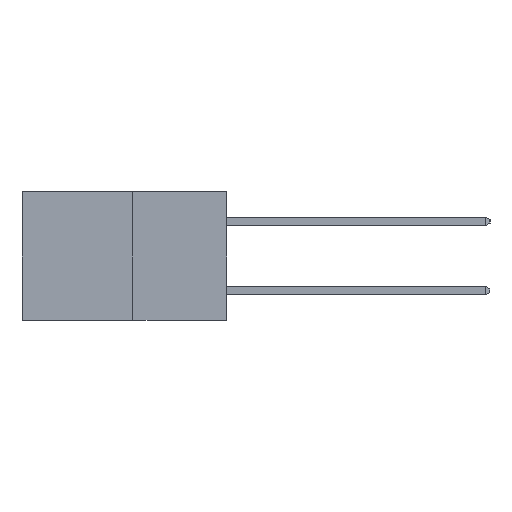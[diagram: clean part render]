
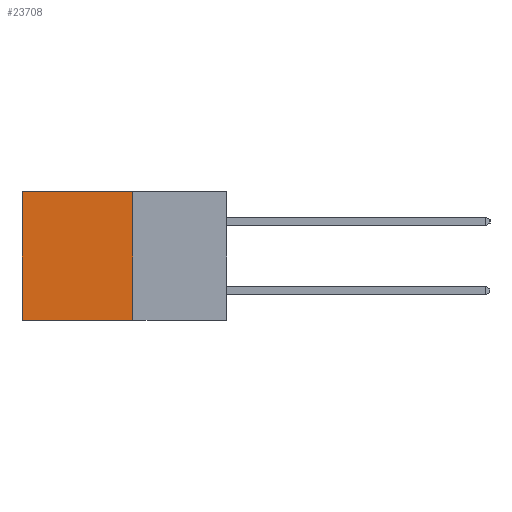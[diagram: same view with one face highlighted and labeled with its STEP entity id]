
A CAD part, left-side view. The second image highlights one B-rep face of the part: STEP entity #23708.
In plain terms, the highlighted planar face has unit normal (-1, 0, 0).
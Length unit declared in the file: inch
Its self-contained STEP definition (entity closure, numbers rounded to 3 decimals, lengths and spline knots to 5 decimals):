
#586 = CARTESIAN_POINT ( 'NONE',  ( 0.277, 0.27, -0.37 ) ) ;
#1063 = DIRECTION ( 'NONE',  ( 0., 1., 0. ) ) ;
#1952 = EDGE_CURVE ( 'NONE', #17042, #14268, #21985, .T. ) ;
#2075 = DIRECTION ( 'NONE',  ( 0., 0., -1. ) ) ;
#2226 = CARTESIAN_POINT ( 'NONE',  ( 0.277, 0.59, -0.37 ) ) ;
#4217 = LINE ( 'NONE', #586, #15182 ) ;
#5504 = EDGE_CURVE ( 'NONE', #17709, #29185, #4217, .T. ) ;
#5731 = CARTESIAN_POINT ( 'NONE',  ( 0.277, 0.27, -0.37 ) ) ;
#6723 = LINE ( 'NONE', #15952, #24613 ) ;
#8320 = CARTESIAN_POINT ( 'NONE',  ( 0.277, 0.59, 0. ) ) ;
#8503 = DIRECTION ( 'NONE',  ( 0., 1., 0. ) ) ;
#9946 = ORIENTED_EDGE ( 'NONE', *, *, #19311, .F. ) ;
#10320 = ORIENTED_EDGE ( 'NONE', *, *, #27218, .T. ) ;
#11307 = CARTESIAN_POINT ( 'NONE',  ( 0.277, 0.27, 0. ) ) ;
#13585 = CARTESIAN_POINT ( 'NONE',  ( 0.277, 0.27, -0.37 ) ) ;
#13895 = AXIS2_PLACEMENT_3D ( 'NONE', #13585, #16037, #2075 ) ;
#14268 = VERTEX_POINT ( 'NONE', #8320 ) ;
#15182 = VECTOR ( 'NONE', #1063, 39.37008 ) ;
#15952 = CARTESIAN_POINT ( 'NONE',  ( 0.277, 0.27, -0.37 ) ) ;
#16037 = DIRECTION ( 'NONE',  ( 1., 0., 0. ) ) ;
#17042 = VERTEX_POINT ( 'NONE', #11307 ) ;
#17619 = EDGE_LOOP ( 'NONE', ( #10320, #29735, #9946, #27621 ) ) ;
#17709 = VERTEX_POINT ( 'NONE', #5731 ) ;
#18183 = LINE ( 'NONE', #2226, #18936 ) ;
#18804 = CARTESIAN_POINT ( 'NONE',  ( 0.277, 0.59, -0.37 ) ) ;
#18936 = VECTOR ( 'NONE', #27805, 39.37008 ) ;
#19311 = EDGE_CURVE ( 'NONE', #17042, #17709, #6723, .T. ) ;
#20399 = CARTESIAN_POINT ( 'NONE',  ( 0.277, 0.27, 0. ) ) ;
#20494 = VECTOR ( 'NONE', #8503, 39.37008 ) ;
#21985 = LINE ( 'NONE', #20399, #20494 ) ;
#23708 = ADVANCED_FACE ( 'NONE', ( #26323 ), #25277, .F. ) ;
#24613 = VECTOR ( 'NONE', #29854, 39.37008 ) ;
#25277 = PLANE ( 'NONE',  #13895 ) ;
#26323 = FACE_OUTER_BOUND ( 'NONE', #17619, .T. ) ;
#27218 = EDGE_CURVE ( 'NONE', #14268, #29185, #18183, .T. ) ;
#27621 = ORIENTED_EDGE ( 'NONE', *, *, #1952, .T. ) ;
#27805 = DIRECTION ( 'NONE',  ( 0., 0., -1. ) ) ;
#29185 = VERTEX_POINT ( 'NONE', #18804 ) ;
#29735 = ORIENTED_EDGE ( 'NONE', *, *, #5504, .F. ) ;
#29854 = DIRECTION ( 'NONE',  ( 0., 0., -1. ) ) ;
